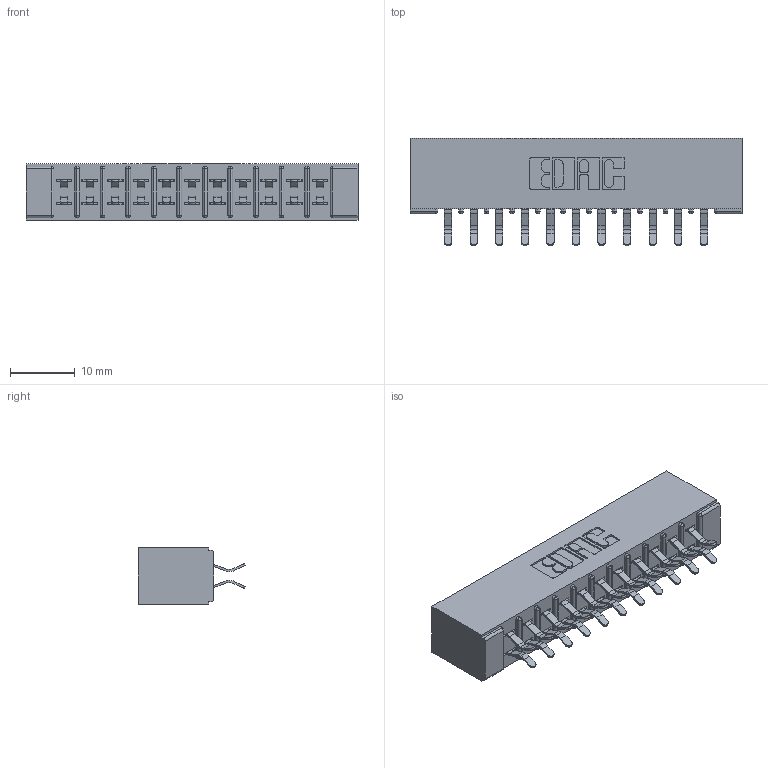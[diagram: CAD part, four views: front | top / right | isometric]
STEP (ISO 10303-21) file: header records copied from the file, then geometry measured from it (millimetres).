
FILE_DESCRIPTION (( 'STEP AP203' ), '1' );
FILE_NAME ('305-022-556-501.STEP', '2019-09-09T13:54:09', ( '' ), ( '' ), 'SwSTEP 2.0', 'SolidWorks 2016', '' );
FILE_SCHEMA (( 'CONFIG_CONTROL_DESIGN' ));
Length unit declared in the file: inch
Products named in the file (3): 305-290-001_556; 305 Part_No Mounting; 305-022-556-501
Assembly tree (23 placements, depth 2):
  305-022-556-501
    305 Part_No Mounting
    305-290-001_556  x22
Bounding box: 51.46 x 16.64 x 8.71 mm (x, y, z)
Volume: 3272.3 mm3; surface area: 6465.9 mm2
Topology: 23 solids, 23 shells, 1340 faces, 3845 edges, 2502 vertices
Faces by surface type: plane 746, cylinder 550, sphere 44
Entity records: 15628 total; most frequent: CARTESIAN_POINT 2587, ORIENTED_EDGE 2562, DIRECTION 2529, EDGE_CURVE 1281, VECTOR 1001, LINE 1001, VERTEX_POINT 822, AXIS2_PLACEMENT_3D 764
